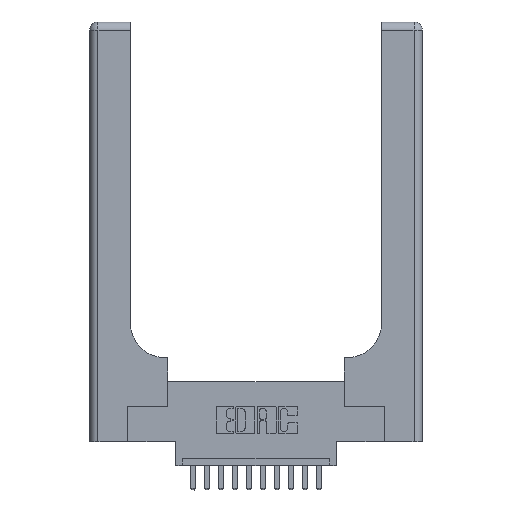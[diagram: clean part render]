
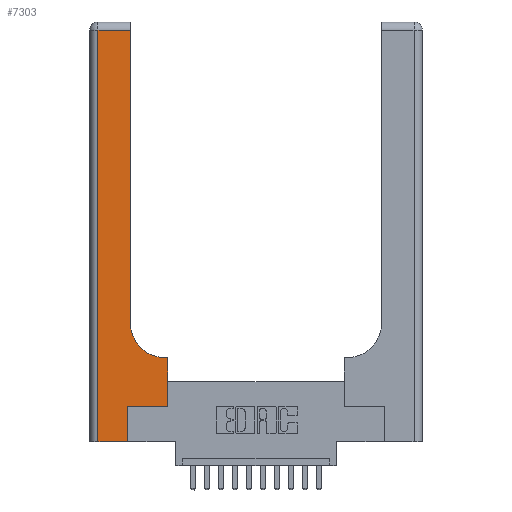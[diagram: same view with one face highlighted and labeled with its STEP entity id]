
A CAD part, top view. The second image highlights one B-rep face of the part: STEP entity #7303.
In plain terms, the highlighted planar face has unit normal (0, 0, 1).
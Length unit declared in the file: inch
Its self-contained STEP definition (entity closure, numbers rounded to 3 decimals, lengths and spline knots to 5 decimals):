
#88 = ORIENTED_EDGE ( 'NONE', *, *, #3922, .T. ) ;
#168 = PLANE ( 'NONE',  #11857 ) ;
#340 = VECTOR ( 'NONE', #12663, 39.37008 ) ;
#489 = CARTESIAN_POINT ( 'NONE',  ( 0.2915, 2.94, 0.37 ) ) ;
#535 = VECTOR ( 'NONE', #16804, 39.37008 ) ;
#857 = EDGE_CURVE ( 'NONE', #14511, #11235, #6608, .T. ) ;
#869 = ORIENTED_EDGE ( 'NONE', *, *, #7227, .T. ) ;
#1083 = CARTESIAN_POINT ( 'NONE',  ( 0.269, 0.25, 0.37 ) ) ;
#1314 = EDGE_CURVE ( 'NONE', #15000, #15222, #2439, .T. ) ;
#1826 = LINE ( 'NONE', #15488, #535 ) ;
#2439 = LINE ( 'NONE', #6766, #4100 ) ;
#2785 = LINE ( 'NONE', #12466, #12547 ) ;
#3476 = VECTOR ( 'NONE', #13569, 39.37008 ) ;
#3628 = VERTEX_POINT ( 'NONE', #13174 ) ;
#3766 = AXIS2_PLACEMENT_3D ( 'NONE', #15596, #6548, #14671 ) ;
#3777 = CIRCLE ( 'NONE', #3766, 0.25 ) ;
#3817 = DIRECTION ( 'NONE',  ( 0., -1., 0. ) ) ;
#3922 = EDGE_CURVE ( 'NONE', #9575, #14511, #11816, .T. ) ;
#4100 = VECTOR ( 'NONE', #13246, 39.37008 ) ;
#4379 = DIRECTION ( 'NONE',  ( 0., 1., 0. ) ) ;
#4721 = ORIENTED_EDGE ( 'NONE', *, *, #10613, .T. ) ;
#4918 = ORIENTED_EDGE ( 'NONE', *, *, #13498, .T. ) ;
#5248 = ORIENTED_EDGE ( 'NONE', *, *, #1314, .T. ) ;
#5620 = ORIENTED_EDGE ( 'NONE', *, *, #7438, .T. ) ;
#6033 = EDGE_CURVE ( 'NONE', #15222, #3628, #2785, .T. ) ;
#6054 = FACE_OUTER_BOUND ( 'NONE', #9627, .T. ) ;
#6374 = CARTESIAN_POINT ( 'NONE',  ( 0.269, 0., 0.37 ) ) ;
#6548 = DIRECTION ( 'NONE',  ( 0., 0., -1. ) ) ;
#6608 = LINE ( 'NONE', #7291, #340 ) ;
#6766 = CARTESIAN_POINT ( 'NONE',  ( 0., 0., 0.37 ) ) ;
#7227 = EDGE_CURVE ( 'NONE', #7862, #15000, #10400, .T. ) ;
#7291 = CARTESIAN_POINT ( 'NONE',  ( 0.2915, 0.6, 0.37 ) ) ;
#7303 = ADVANCED_FACE ( 'NONE', ( #6054 ), #168, .F. ) ;
#7438 = EDGE_CURVE ( 'NONE', #11558, #7862, #12081, .T. ) ;
#7823 = CARTESIAN_POINT ( 'NONE',  ( 0.2915, 0.85, 0.37 ) ) ;
#7862 = VERTEX_POINT ( 'NONE', #10743 ) ;
#8944 = VERTEX_POINT ( 'NONE', #7823 ) ;
#8997 = CARTESIAN_POINT ( 'NONE',  ( 0.06, 3., 0.37 ) ) ;
#9249 = EDGE_CURVE ( 'NONE', #3628, #9575, #11753, .T. ) ;
#9363 = VECTOR ( 'NONE', #12207, 39.37008 ) ;
#9564 = DIRECTION ( 'NONE',  ( -1., 0., 0. ) ) ;
#9575 = VERTEX_POINT ( 'NONE', #11494 ) ;
#9627 = EDGE_LOOP ( 'NONE', ( #4918, #5620, #869, #5248, #17000, #12311, #88, #11319, #4721 ) ) ;
#10400 = LINE ( 'NONE', #8997, #13561 ) ;
#10613 = EDGE_CURVE ( 'NONE', #11235, #8944, #3777, .T. ) ;
#10712 = CARTESIAN_POINT ( 'NONE',  ( 0., 3., 0.37 ) ) ;
#10743 = CARTESIAN_POINT ( 'NONE',  ( 0.06, 2.94, 0.37 ) ) ;
#10772 = DIRECTION ( 'NONE',  ( 0., 0., -1. ) ) ;
#11235 = VERTEX_POINT ( 'NONE', #12451 ) ;
#11319 = ORIENTED_EDGE ( 'NONE', *, *, #857, .T. ) ;
#11494 = CARTESIAN_POINT ( 'NONE',  ( 0.5585, 0.25, 0.37 ) ) ;
#11558 = VERTEX_POINT ( 'NONE', #489 ) ;
#11753 = LINE ( 'NONE', #1083, #13000 ) ;
#11816 = LINE ( 'NONE', #15018, #3476 ) ;
#11857 = AXIS2_PLACEMENT_3D ( 'NONE', #10712, #10772, #9564 ) ;
#12081 = LINE ( 'NONE', #13649, #9363 ) ;
#12207 = DIRECTION ( 'NONE',  ( -1., 0., 0. ) ) ;
#12311 = ORIENTED_EDGE ( 'NONE', *, *, #9249, .T. ) ;
#12451 = CARTESIAN_POINT ( 'NONE',  ( 0.5415, 0.6, 0.37 ) ) ;
#12466 = CARTESIAN_POINT ( 'NONE',  ( 0.269, 0., 0.37 ) ) ;
#12547 = VECTOR ( 'NONE', #4379, 39.37008 ) ;
#12663 = DIRECTION ( 'NONE',  ( -1., 0., 0. ) ) ;
#13000 = VECTOR ( 'NONE', #15782, 39.37008 ) ;
#13174 = CARTESIAN_POINT ( 'NONE',  ( 0.269, 0.25, 0.37 ) ) ;
#13246 = DIRECTION ( 'NONE',  ( 1., 0., 0. ) ) ;
#13498 = EDGE_CURVE ( 'NONE', #8944, #11558, #1826, .T. ) ;
#13561 = VECTOR ( 'NONE', #3817, 39.37008 ) ;
#13569 = DIRECTION ( 'NONE',  ( 0., 1., 0. ) ) ;
#13649 = CARTESIAN_POINT ( 'NONE',  ( 0., 2.94, 0.37 ) ) ;
#13749 = CARTESIAN_POINT ( 'NONE',  ( 0.06, 0., 0.37 ) ) ;
#14511 = VERTEX_POINT ( 'NONE', #15218 ) ;
#14671 = DIRECTION ( 'NONE',  ( 1., 0., 0. ) ) ;
#15000 = VERTEX_POINT ( 'NONE', #13749 ) ;
#15018 = CARTESIAN_POINT ( 'NONE',  ( 0.5585, 0.25, 0.37 ) ) ;
#15218 = CARTESIAN_POINT ( 'NONE',  ( 0.5585, 0.6, 0.37 ) ) ;
#15222 = VERTEX_POINT ( 'NONE', #6374 ) ;
#15488 = CARTESIAN_POINT ( 'NONE',  ( 0.2915, 3., 0.37 ) ) ;
#15596 = CARTESIAN_POINT ( 'NONE',  ( 0.5415, 0.85, 0.37 ) ) ;
#15782 = DIRECTION ( 'NONE',  ( 1., 0., 0. ) ) ;
#16804 = DIRECTION ( 'NONE',  ( 0., 1., 0. ) ) ;
#17000 = ORIENTED_EDGE ( 'NONE', *, *, #6033, .T. ) ;
